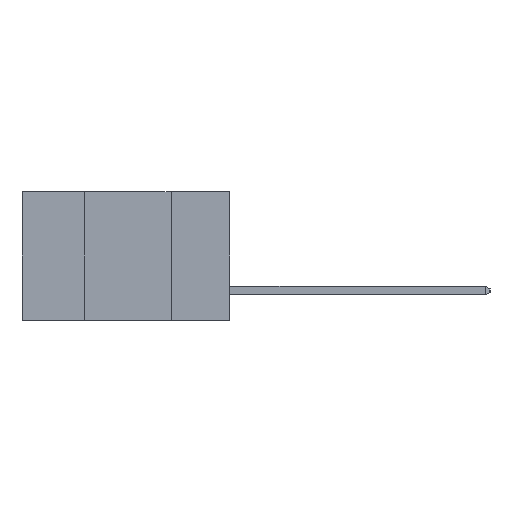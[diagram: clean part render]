
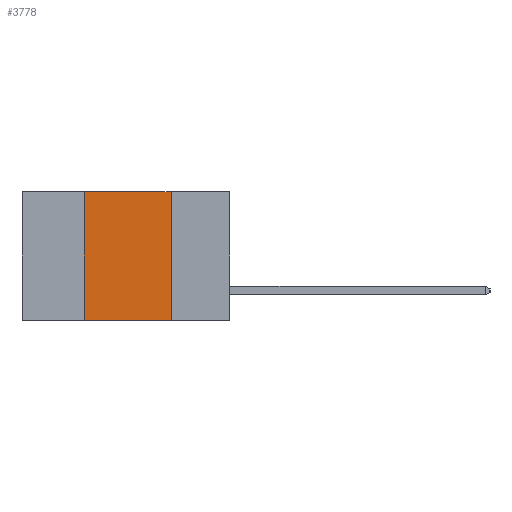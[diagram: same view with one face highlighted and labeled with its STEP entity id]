
A CAD part, left-side view. The second image highlights one B-rep face of the part: STEP entity #3778.
In plain terms, the highlighted planar face has unit normal (-1, 0, 0).
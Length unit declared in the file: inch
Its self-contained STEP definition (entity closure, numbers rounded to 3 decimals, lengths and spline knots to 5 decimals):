
#43 = DIRECTION ( 'NONE',  ( 0., -1., 0. ) ) ;
#66 = EDGE_CURVE ( 'NONE', #573, #1623, #179, .T. ) ;
#176 = CARTESIAN_POINT ( 'NONE',  ( 0., 0.6, 0. ) ) ;
#179 = LINE ( 'NONE', #12040, #7353 ) ;
#573 = VERTEX_POINT ( 'NONE', #11164 ) ;
#855 = CARTESIAN_POINT ( 'NONE',  ( 0., 0.42, 0. ) ) ;
#928 = CARTESIAN_POINT ( 'NONE',  ( 0., 0.17, 0. ) ) ;
#950 = ORIENTED_EDGE ( 'NONE', *, *, #10656, .F. ) ;
#1088 = LINE ( 'NONE', #8005, #8602 ) ;
#1294 = LINE ( 'NONE', #10916, #8787 ) ;
#1363 = FACE_OUTER_BOUND ( 'NONE', #3872, .T. ) ;
#1623 = VERTEX_POINT ( 'NONE', #8836 ) ;
#2012 = DIRECTION ( 'NONE',  ( 0., 0., -1. ) ) ;
#2514 = VECTOR ( 'NONE', #2012, 39.37008 ) ;
#3778 = ADVANCED_FACE ( 'NONE', ( #1363 ), #4934, .F. ) ;
#3872 = EDGE_LOOP ( 'NONE', ( #5688, #950, #11240, #11816 ) ) ;
#4934 = PLANE ( 'NONE',  #8369 ) ;
#5688 = ORIENTED_EDGE ( 'NONE', *, *, #8572, .F. ) ;
#6531 = VERTEX_POINT ( 'NONE', #855 ) ;
#7159 = VERTEX_POINT ( 'NONE', #11340 ) ;
#7353 = VECTOR ( 'NONE', #43, 39.37008 ) ;
#7592 = EDGE_CURVE ( 'NONE', #573, #6531, #1088, .T. ) ;
#8005 = CARTESIAN_POINT ( 'NONE',  ( 0., 0.42, 0. ) ) ;
#8369 = AXIS2_PLACEMENT_3D ( 'NONE', #176, #8977, #9897 ) ;
#8572 = EDGE_CURVE ( 'NONE', #7159, #1623, #12460, .T. ) ;
#8602 = VECTOR ( 'NONE', #9026, 39.37008 ) ;
#8787 = VECTOR ( 'NONE', #11892, 39.37008 ) ;
#8836 = CARTESIAN_POINT ( 'NONE',  ( 0., 0.17, -0.37 ) ) ;
#8977 = DIRECTION ( 'NONE',  ( 1., 0., 0. ) ) ;
#9026 = DIRECTION ( 'NONE',  ( 0., 0., 1. ) ) ;
#9897 = DIRECTION ( 'NONE',  ( 0., 0., -1. ) ) ;
#10656 = EDGE_CURVE ( 'NONE', #6531, #7159, #1294, .T. ) ;
#10916 = CARTESIAN_POINT ( 'NONE',  ( 0., 0.6, 0. ) ) ;
#11164 = CARTESIAN_POINT ( 'NONE',  ( 0., 0.42, -0.37 ) ) ;
#11240 = ORIENTED_EDGE ( 'NONE', *, *, #7592, .F. ) ;
#11340 = CARTESIAN_POINT ( 'NONE',  ( 0., 0.17, 0. ) ) ;
#11816 = ORIENTED_EDGE ( 'NONE', *, *, #66, .T. ) ;
#11892 = DIRECTION ( 'NONE',  ( 0., -1., 0. ) ) ;
#12040 = CARTESIAN_POINT ( 'NONE',  ( 0., 0.6, -0.37 ) ) ;
#12460 = LINE ( 'NONE', #928, #2514 ) ;
